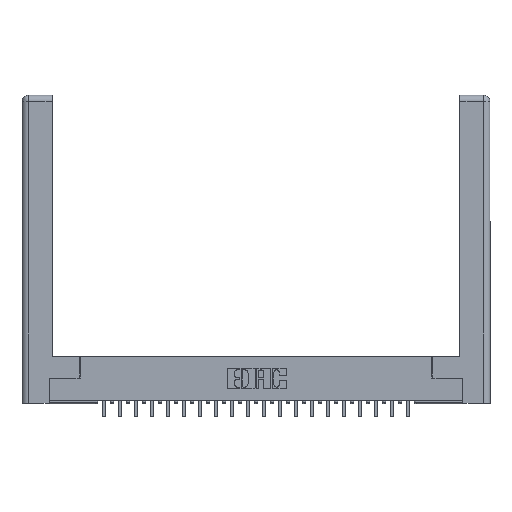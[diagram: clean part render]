
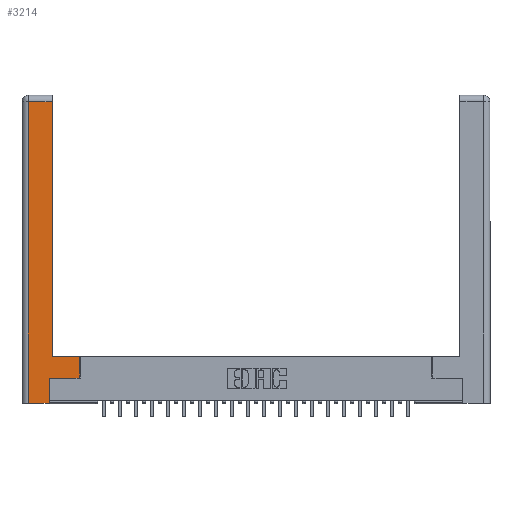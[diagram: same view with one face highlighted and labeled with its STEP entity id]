
A CAD part, top view. The second image highlights one B-rep face of the part: STEP entity #3214.
In plain terms, the highlighted planar face has unit normal (0, 0, 1).
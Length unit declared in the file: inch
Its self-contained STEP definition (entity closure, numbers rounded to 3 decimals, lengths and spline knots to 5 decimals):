
#198 = ORIENTED_EDGE ( 'NONE', *, *, #13974, .T. ) ;
#413 = ORIENTED_EDGE ( 'NONE', *, *, #10253, .T. ) ;
#434 = ORIENTED_EDGE ( 'NONE', *, *, #5619, .T. ) ;
#636 = ORIENTED_EDGE ( 'NONE', *, *, #10533, .T. ) ;
#680 = ORIENTED_EDGE ( 'NONE', *, *, #6374, .T. ) ;
#816 = VERTEX_POINT ( 'NONE', #9278 ) ;
#823 = ORIENTED_EDGE ( 'NONE', *, *, #2601, .T. ) ;
#875 = CARTESIAN_POINT ( 'NONE',  ( 0.295, 3., 0. ) ) ;
#982 = CARTESIAN_POINT ( 'NONE',  ( 0., 0., 0. ) ) ;
#1209 = VERTEX_POINT ( 'NONE', #3990 ) ;
#1297 = ORIENTED_EDGE ( 'NONE', *, *, #22596, .T. ) ;
#1689 = CARTESIAN_POINT ( 'NONE',  ( 0.265, 0., 0. ) ) ;
#2601 = EDGE_CURVE ( 'NONE', #816, #19806, #19985, .T. ) ;
#2917 = DIRECTION ( 'NONE',  ( 0., 0., -1. ) ) ;
#2934 = VECTOR ( 'NONE', #10067, 39.37008 ) ;
#3214 = ADVANCED_FACE ( 'NONE', ( #20811 ), #14105, .F. ) ;
#3518 = LINE ( 'NONE', #22952, #2934 ) ;
#3880 = DIRECTION ( 'NONE',  ( 0., 1., 0. ) ) ;
#3990 = CARTESIAN_POINT ( 'NONE',  ( 0.295, 2.94, 0. ) ) ;
#4435 = CARTESIAN_POINT ( 'NONE',  ( 0.0615, 2.94, 0. ) ) ;
#5052 = LINE ( 'NONE', #1689, #5657 ) ;
#5084 = CARTESIAN_POINT ( 'NONE',  ( 0.265, 0., 0. ) ) ;
#5619 = EDGE_CURVE ( 'NONE', #16287, #19785, #8521, .T. ) ;
#5657 = VECTOR ( 'NONE', #20277, 39.37008 ) ;
#5824 = CARTESIAN_POINT ( 'NONE',  ( 0.565, 0.45, 0. ) ) ;
#5868 = LINE ( 'NONE', #5824, #10764 ) ;
#5979 = VERTEX_POINT ( 'NONE', #15801 ) ;
#6374 = EDGE_CURVE ( 'NONE', #23771, #816, #5868, .T. ) ;
#8212 = CARTESIAN_POINT ( 'NONE',  ( 0.295, 0.45, 0. ) ) ;
#8431 = CARTESIAN_POINT ( 'NONE',  ( 0.265, 0.245, 0. ) ) ;
#8521 = LINE ( 'NONE', #8431, #17763 ) ;
#9278 = CARTESIAN_POINT ( 'NONE',  ( 0.565, 0.45, 0. ) ) ;
#9343 = CARTESIAN_POINT ( 'NONE',  ( 0.295, 0.45, 0. ) ) ;
#9563 = VECTOR ( 'NONE', #20659, 39.37008 ) ;
#9628 = CARTESIAN_POINT ( 'NONE',  ( 0.0615, 2.94, 0. ) ) ;
#10067 = DIRECTION ( 'NONE',  ( 1., 0., 0. ) ) ;
#10253 = EDGE_CURVE ( 'NONE', #5979, #16287, #5052, .T. ) ;
#10302 = CARTESIAN_POINT ( 'NONE',  ( 0.565, 0.245, 0. ) ) ;
#10453 = VECTOR ( 'NONE', #15882, 39.37008 ) ;
#10510 = VERTEX_POINT ( 'NONE', #4435 ) ;
#10533 = EDGE_CURVE ( 'NONE', #19785, #23771, #3518, .T. ) ;
#10656 = LINE ( 'NONE', #18779, #23612 ) ;
#10764 = VECTOR ( 'NONE', #3880, 39.37008 ) ;
#11459 = DIRECTION ( 'NONE',  ( -1., 0., 0. ) ) ;
#11600 = LINE ( 'NONE', #875, #10453 ) ;
#11993 = EDGE_LOOP ( 'NONE', ( #18677, #1297, #198, #413, #434, #636, #680, #823 ) ) ;
#12327 = EDGE_CURVE ( 'NONE', #19806, #1209, #11600, .T. ) ;
#13241 = DIRECTION ( 'NONE',  ( 0., -1., 0. ) ) ;
#13974 = EDGE_CURVE ( 'NONE', #10510, #5979, #10656, .T. ) ;
#14105 = PLANE ( 'NONE',  #22082 ) ;
#15801 = CARTESIAN_POINT ( 'NONE',  ( 0.0615, 0., 0. ) ) ;
#15882 = DIRECTION ( 'NONE',  ( 0., 1., 0. ) ) ;
#15984 = DIRECTION ( 'NONE',  ( -1., 0., 0. ) ) ;
#16287 = VERTEX_POINT ( 'NONE', #5084 ) ;
#17338 = CARTESIAN_POINT ( 'NONE',  ( 0.265, 0.245, 0. ) ) ;
#17763 = VECTOR ( 'NONE', #23147, 39.37008 ) ;
#18677 = ORIENTED_EDGE ( 'NONE', *, *, #12327, .T. ) ;
#18779 = CARTESIAN_POINT ( 'NONE',  ( 0.0615, 0., 0. ) ) ;
#18905 = VECTOR ( 'NONE', #11459, 39.37008 ) ;
#19785 = VERTEX_POINT ( 'NONE', #17338 ) ;
#19806 = VERTEX_POINT ( 'NONE', #8212 ) ;
#19985 = LINE ( 'NONE', #9343, #9563 ) ;
#20277 = DIRECTION ( 'NONE',  ( 1., 0., 0. ) ) ;
#20659 = DIRECTION ( 'NONE',  ( -1., 0., 0. ) ) ;
#20811 = FACE_OUTER_BOUND ( 'NONE', #11993, .T. ) ;
#22082 = AXIS2_PLACEMENT_3D ( 'NONE', #982, #2917, #15984 ) ;
#22596 = EDGE_CURVE ( 'NONE', #1209, #10510, #23178, .T. ) ;
#22952 = CARTESIAN_POINT ( 'NONE',  ( 0.565, 0.245, 0. ) ) ;
#23147 = DIRECTION ( 'NONE',  ( 0., 1., 0. ) ) ;
#23178 = LINE ( 'NONE', #9628, #18905 ) ;
#23612 = VECTOR ( 'NONE', #13241, 39.37008 ) ;
#23771 = VERTEX_POINT ( 'NONE', #10302 ) ;
